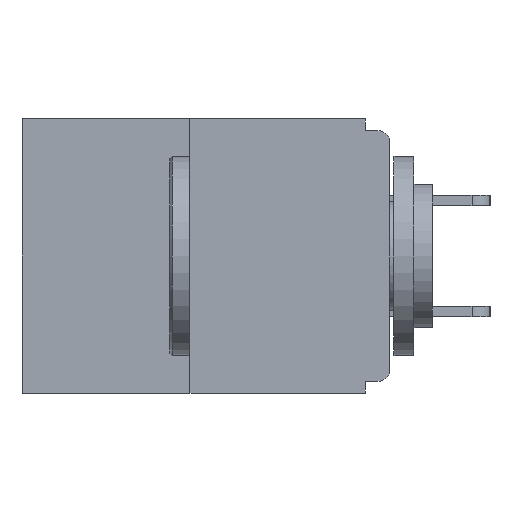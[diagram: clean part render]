
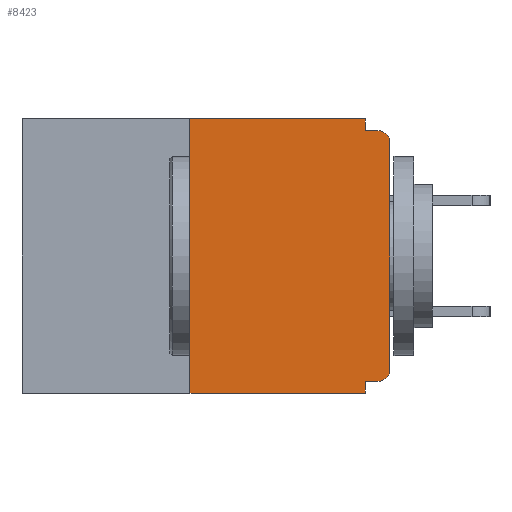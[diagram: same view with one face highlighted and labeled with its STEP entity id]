
A CAD part, left-side view. The second image highlights one B-rep face of the part: STEP entity #8423.
In plain terms, the highlighted planar face has unit normal (-1, 0, 0).
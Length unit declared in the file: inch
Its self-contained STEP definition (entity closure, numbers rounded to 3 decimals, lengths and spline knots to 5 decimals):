
#152 = VECTOR ( 'NONE', #10077, 39.37008 ) ;
#479 = CARTESIAN_POINT ( 'NONE',  ( 0., 0.015, -0.03 ) ) ;
#838 = CARTESIAN_POINT ( 'NONE',  ( 0., 0.031, -0.343 ) ) ;
#1333 = CARTESIAN_POINT ( 'NONE',  ( 0., 0., 0. ) ) ;
#1387 = ORIENTED_EDGE ( 'NONE', *, *, #10710, .F. ) ;
#1494 = CARTESIAN_POINT ( 'NONE',  ( 0., 0.031, 0. ) ) ;
#1935 = EDGE_CURVE ( 'NONE', #17820, #6814, #20633, .T. ) ;
#2331 = EDGE_CURVE ( 'NONE', #17820, #9896, #4071, .T. ) ;
#2402 = VERTEX_POINT ( 'NONE', #17261 ) ;
#2577 = VERTEX_POINT ( 'NONE', #6223 ) ;
#2785 = ORIENTED_EDGE ( 'NONE', *, *, #15752, .F. ) ;
#3071 = ORIENTED_EDGE ( 'NONE', *, *, #11693, .T. ) ;
#3322 = CARTESIAN_POINT ( 'NONE',  ( 0., 0., -0.03 ) ) ;
#3375 = DIRECTION ( 'NONE',  ( 0., 0., -1. ) ) ;
#3397 = DIRECTION ( 'NONE',  ( 0., 0., -1. ) ) ;
#3656 = CIRCLE ( 'NONE', #6059, 0.015 ) ;
#3680 = DIRECTION ( 'NONE',  ( 0., 0., -1. ) ) ;
#4071 = LINE ( 'NONE', #9772, #152 ) ;
#4161 = CARTESIAN_POINT ( 'NONE',  ( 0., 0.015, -0.313 ) ) ;
#4710 = CARTESIAN_POINT ( 'NONE',  ( 0., 0.25, 0. ) ) ;
#4969 = LINE ( 'NONE', #1333, #8850 ) ;
#5025 = VERTEX_POINT ( 'NONE', #10151 ) ;
#5727 = VERTEX_POINT ( 'NONE', #1494 ) ;
#6050 = DIRECTION ( 'NONE',  ( 0., -1., 0. ) ) ;
#6059 = AXIS2_PLACEMENT_3D ( 'NONE', #479, #7234, #3680 ) ;
#6223 = CARTESIAN_POINT ( 'NONE',  ( 0., 0.015, -0.015 ) ) ;
#6626 = CARTESIAN_POINT ( 'NONE',  ( 0., 0.031, -0.343 ) ) ;
#6814 = VERTEX_POINT ( 'NONE', #4710 ) ;
#6938 = CARTESIAN_POINT ( 'NONE',  ( 0., 0.46, 0. ) ) ;
#6982 = EDGE_CURVE ( 'NONE', #5727, #2402, #10274, .T. ) ;
#7234 = DIRECTION ( 'NONE',  ( -1., 0., 0. ) ) ;
#7250 = VECTOR ( 'NONE', #3375, 39.37008 ) ;
#7360 = FACE_OUTER_BOUND ( 'NONE', #16866, .T. ) ;
#7470 = LINE ( 'NONE', #21347, #8218 ) ;
#7603 = DIRECTION ( 'NONE',  ( 0., 0., -1. ) ) ;
#7703 = VERTEX_POINT ( 'NONE', #8728 ) ;
#7867 = ORIENTED_EDGE ( 'NONE', *, *, #2331, .T. ) ;
#8123 = CARTESIAN_POINT ( 'NONE',  ( 0., 0.031, -0.328 ) ) ;
#8137 = CARTESIAN_POINT ( 'NONE',  ( 0., 0.25, -0.343 ) ) ;
#8218 = VECTOR ( 'NONE', #16352, 39.37008 ) ;
#8382 = PLANE ( 'NONE',  #12214 ) ;
#8423 = ADVANCED_FACE ( 'NONE', ( #7360 ), #8382, .F. ) ;
#8728 = CARTESIAN_POINT ( 'NONE',  ( 0., 0.015, -0.328 ) ) ;
#8850 = VECTOR ( 'NONE', #14583, 39.37008 ) ;
#9339 = EDGE_CURVE ( 'NONE', #6814, #5727, #15323, .T. ) ;
#9624 = EDGE_CURVE ( 'NONE', #5025, #17144, #4969, .T. ) ;
#9772 = CARTESIAN_POINT ( 'NONE',  ( 0., 0.46, -0.343 ) ) ;
#9782 = VECTOR ( 'NONE', #10117, 39.37008 ) ;
#9896 = VERTEX_POINT ( 'NONE', #838 ) ;
#10077 = DIRECTION ( 'NONE',  ( 0., -1., 0. ) ) ;
#10117 = DIRECTION ( 'NONE',  ( 0., 0., 1. ) ) ;
#10151 = CARTESIAN_POINT ( 'NONE',  ( 0., 0., -0.313 ) ) ;
#10245 = ORIENTED_EDGE ( 'NONE', *, *, #9339, .F. ) ;
#10274 = LINE ( 'NONE', #20881, #15996 ) ;
#10710 = EDGE_CURVE ( 'NONE', #21349, #9896, #12429, .T. ) ;
#11693 = EDGE_CURVE ( 'NONE', #17144, #2577, #3656, .T. ) ;
#11705 = ORIENTED_EDGE ( 'NONE', *, *, #6982, .F. ) ;
#12214 = AXIS2_PLACEMENT_3D ( 'NONE', #6938, #15058, #3397 ) ;
#12429 = LINE ( 'NONE', #6626, #7250 ) ;
#12432 = ORIENTED_EDGE ( 'NONE', *, *, #1935, .F. ) ;
#13146 = EDGE_CURVE ( 'NONE', #7703, #21349, #7470, .T. ) ;
#13516 = VECTOR ( 'NONE', #6050, 39.37008 ) ;
#13809 = CARTESIAN_POINT ( 'NONE',  ( 0., 0., -0.015 ) ) ;
#13927 = DIRECTION ( 'NONE',  ( -1., 0., 0. ) ) ;
#14351 = VECTOR ( 'NONE', #15696, 39.37008 ) ;
#14583 = DIRECTION ( 'NONE',  ( 0., 0., 1. ) ) ;
#14677 = ORIENTED_EDGE ( 'NONE', *, *, #16558, .T. ) ;
#15058 = DIRECTION ( 'NONE',  ( 1., 0., 0. ) ) ;
#15085 = CIRCLE ( 'NONE', #15893, 0.015 ) ;
#15323 = LINE ( 'NONE', #21048, #13516 ) ;
#15696 = DIRECTION ( 'NONE',  ( 0., -1., 0. ) ) ;
#15752 = EDGE_CURVE ( 'NONE', #2402, #2577, #18722, .T. ) ;
#15893 = AXIS2_PLACEMENT_3D ( 'NONE', #4161, #13927, #17209 ) ;
#15996 = VECTOR ( 'NONE', #7603, 39.37008 ) ;
#16352 = DIRECTION ( 'NONE',  ( 0., 1., 0. ) ) ;
#16558 = EDGE_CURVE ( 'NONE', #7703, #5025, #15085, .T. ) ;
#16866 = EDGE_LOOP ( 'NONE', ( #10245, #12432, #7867, #1387, #18875, #14677, #21188, #3071, #2785, #11705 ) ) ;
#17144 = VERTEX_POINT ( 'NONE', #3322 ) ;
#17209 = DIRECTION ( 'NONE',  ( 0., 0., -1. ) ) ;
#17261 = CARTESIAN_POINT ( 'NONE',  ( 0., 0.031, -0.015 ) ) ;
#17820 = VERTEX_POINT ( 'NONE', #8137 ) ;
#18722 = LINE ( 'NONE', #13809, #14351 ) ;
#18875 = ORIENTED_EDGE ( 'NONE', *, *, #13146, .F. ) ;
#19974 = CARTESIAN_POINT ( 'NONE',  ( 0., 0.25, 0. ) ) ;
#20633 = LINE ( 'NONE', #19974, #9782 ) ;
#20881 = CARTESIAN_POINT ( 'NONE',  ( 0., 0.031, 0. ) ) ;
#21048 = CARTESIAN_POINT ( 'NONE',  ( 0., 0.46, 0. ) ) ;
#21188 = ORIENTED_EDGE ( 'NONE', *, *, #9624, .T. ) ;
#21347 = CARTESIAN_POINT ( 'NONE',  ( 0., 0., -0.328 ) ) ;
#21349 = VERTEX_POINT ( 'NONE', #8123 ) ;
